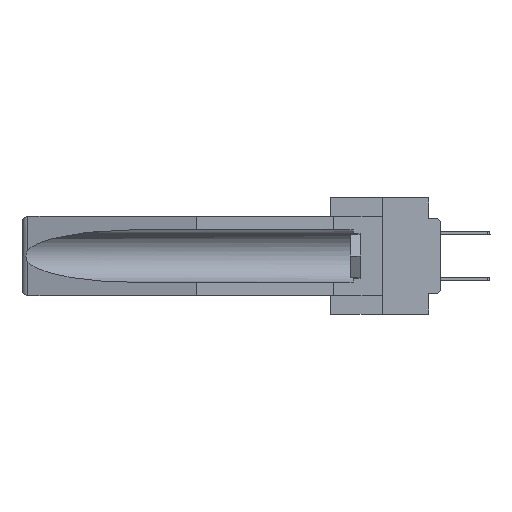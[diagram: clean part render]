
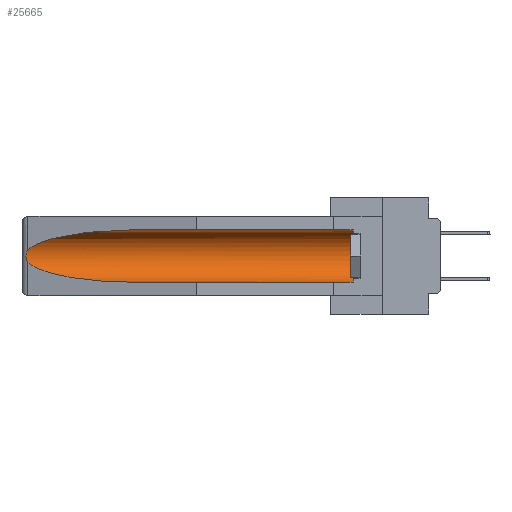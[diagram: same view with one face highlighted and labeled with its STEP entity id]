
A CAD part, left-side view. The second image highlights one B-rep face of the part: STEP entity #25665.
In plain terms, the highlighted cylindrical face has radius 2.857 mm (diameter 5.715 mm), a partial arc.
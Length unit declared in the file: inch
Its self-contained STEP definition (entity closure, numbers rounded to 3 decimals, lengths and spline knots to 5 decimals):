
#781 = DIRECTION ( 'NONE',  ( 0., 1., 0. ) ) ;
#2296 = B_SPLINE_CURVE_WITH_KNOTS ( 'NONE', 3,
 ( #31981, #20603, #7897, #35157, #5261, #5148, #26919, #10725, #21651, #21196 ),
 .UNSPECIFIED., .F., .F.,
 ( 4, 2, 2, 2, 4 ),
 ( 0., 0.00029, 0.00058, 0.00087, 0.00117 ),
 .UNSPECIFIED. ) ;
#3441 = CARTESIAN_POINT ( 'NONE',  ( 0.26537, 1.52718, -0.19328 ) ) ;
#3560 = CARTESIAN_POINT ( 'NONE',  ( 0.21114, 1.30732, -0.284 ) ) ;
#3565 = LINE ( 'NONE', #33325, #16690 ) ;
#5086 = VERTEX_POINT ( 'NONE', #35003 ) ;
#5148 = CARTESIAN_POINT ( 'NONE',  ( 0.2675, 1.53308, -0.17534 ) ) ;
#5261 = CARTESIAN_POINT ( 'NONE',  ( 0.2675, 1.53308, -0.16763 ) ) ;
#6193 = CARTESIAN_POINT ( 'NONE',  ( 0.25451, 1.48313, -0.24835 ) ) ;
#6838 = CARTESIAN_POINT ( 'NONE',  ( 0.155, 0.126, -0.1715 ) ) ;
#7038 = DIRECTION ( 'NONE',  ( 0., 1., 0. ) ) ;
#7275 = DIRECTION ( 'NONE',  ( 0., 0., 1. ) ) ;
#7372 = CARTESIAN_POINT ( 'NONE',  ( 0.26537, 1.52718, -0.19328 ) ) ;
#7897 = CARTESIAN_POINT ( 'NONE',  ( 0.26654, 1.53092, -0.15636 ) ) ;
#8513 = VERTEX_POINT ( 'NONE', #11826 ) ;
#10003 = CIRCLE ( 'NONE', #25782, 0.1125 ) ;
#10067 = ORIENTED_EDGE ( 'NONE', *, *, #34337, .T. ) ;
#10092 = CARTESIAN_POINT ( 'NONE',  ( 0.155, -0.30754, -0.1715 ) ) ;
#10140 = VECTOR ( 'NONE', #12170, 39.37008 ) ;
#10193 =( BOUNDED_CURVE ( )  B_SPLINE_CURVE ( 3, ( #3441, #6193, #3560, #12020 ),
 .UNSPECIFIED., .F., .F. ) 
 B_SPLINE_CURVE_WITH_KNOTS ( ( 4, 4 ),
 ( 0.1948, 1.5708 ),
 .UNSPECIFIED. ) 
 CURVE ( )  GEOMETRIC_REPRESENTATION_ITEM ( )  RATIONAL_B_SPLINE_CURVE ( ( 1., 0.848, 0.848, 1. ) ) 
 REPRESENTATION_ITEM ( '' )  );
#10725 = CARTESIAN_POINT ( 'NONE',  ( 0.26655, 1.53094, -0.18657 ) ) ;
#11826 = CARTESIAN_POINT ( 'NONE',  ( 0.155, 1.07973, -0.059 ) ) ;
#12020 = CARTESIAN_POINT ( 'NONE',  ( 0.155, 1.07973, -0.284 ) ) ;
#12170 = DIRECTION ( 'NONE',  ( 0., 1., 0. ) ) ;
#12618 = EDGE_LOOP ( 'NONE', ( #10067, #15345, #19010, #19520, #24973, #12813 ) ) ;
#12813 = ORIENTED_EDGE ( 'NONE', *, *, #26902, .T. ) ;
#13822 =( BOUNDED_CURVE ( )  B_SPLINE_CURVE ( 3, ( #18203, #20473, #28672, #17851 ),
 .UNSPECIFIED., .F., .F. ) 
 B_SPLINE_CURVE_WITH_KNOTS ( ( 4, 4 ),
 ( 4.71239, 6.08839 ),
 .UNSPECIFIED. ) 
 CURVE ( )  GEOMETRIC_REPRESENTATION_ITEM ( )  RATIONAL_B_SPLINE_CURVE ( ( 1., 0.848, 0.848, 1. ) ) 
 REPRESENTATION_ITEM ( '' )  );
#13954 = EDGE_CURVE ( 'NONE', #5086, #28427, #10003, .T. ) ;
#14765 = VERTEX_POINT ( 'NONE', #23408 ) ;
#14790 = LINE ( 'NONE', #26214, #10140 ) ;
#15345 = ORIENTED_EDGE ( 'NONE', *, *, #29674, .T. ) ;
#16668 = FACE_OUTER_BOUND ( 'NONE', #12618, .T. ) ;
#16690 = VECTOR ( 'NONE', #781, 39.37008 ) ;
#16967 = CARTESIAN_POINT ( 'NONE',  ( 0.155, 1.07973, -0.284 ) ) ;
#17052 = DIRECTION ( 'NONE',  ( 0., 0., 1. ) ) ;
#17851 = CARTESIAN_POINT ( 'NONE',  ( 0.26537, 1.52718, -0.14972 ) ) ;
#17987 = CYLINDRICAL_SURFACE ( 'NONE', #22239, 0.1125 ) ;
#18203 = CARTESIAN_POINT ( 'NONE',  ( 0.155, 1.07973, -0.059 ) ) ;
#19010 = ORIENTED_EDGE ( 'NONE', *, *, #29144, .T. ) ;
#19520 = ORIENTED_EDGE ( 'NONE', *, *, #32947, .F. ) ;
#20473 = CARTESIAN_POINT ( 'NONE',  ( 0.21114, 1.30732, -0.059 ) ) ;
#20603 = CARTESIAN_POINT ( 'NONE',  ( 0.26597, 1.52961, -0.15275 ) ) ;
#21196 = CARTESIAN_POINT ( 'NONE',  ( 0.26537, 1.52718, -0.19328 ) ) ;
#21651 = CARTESIAN_POINT ( 'NONE',  ( 0.26597, 1.5296, -0.19026 ) ) ;
#22239 = AXIS2_PLACEMENT_3D ( 'NONE', #10092, #7038, #7275 ) ;
#22422 = DIRECTION ( 'NONE',  ( 0., -1., 0. ) ) ;
#23408 = CARTESIAN_POINT ( 'NONE',  ( 0.26537, 1.52718, -0.14972 ) ) ;
#24973 = ORIENTED_EDGE ( 'NONE', *, *, #13954, .T. ) ;
#25665 = ADVANCED_FACE ( 'NONE', ( #16668 ), #17987, .F. ) ;
#25782 = AXIS2_PLACEMENT_3D ( 'NONE', #6838, #22422, #17052 ) ;
#26214 = CARTESIAN_POINT ( 'NONE',  ( 0.155, -0.30754, -0.059 ) ) ;
#26902 = EDGE_CURVE ( 'NONE', #28427, #8513, #14790, .T. ) ;
#26919 = CARTESIAN_POINT ( 'NONE',  ( 0.2673, 1.53269, -0.17917 ) ) ;
#27284 = VERTEX_POINT ( 'NONE', #16967 ) ;
#28427 = VERTEX_POINT ( 'NONE', #35076 ) ;
#28672 = CARTESIAN_POINT ( 'NONE',  ( 0.25451, 1.48313, -0.09465 ) ) ;
#29144 = EDGE_CURVE ( 'NONE', #29353, #27284, #10193, .T. ) ;
#29353 = VERTEX_POINT ( 'NONE', #7372 ) ;
#29674 = EDGE_CURVE ( 'NONE', #14765, #29353, #2296, .T. ) ;
#31981 = CARTESIAN_POINT ( 'NONE',  ( 0.26537, 1.52718, -0.14972 ) ) ;
#32947 = EDGE_CURVE ( 'NONE', #5086, #27284, #3565, .T. ) ;
#33325 = CARTESIAN_POINT ( 'NONE',  ( 0.155, -0.30754, -0.284 ) ) ;
#34337 = EDGE_CURVE ( 'NONE', #8513, #14765, #13822, .T. ) ;
#35003 = CARTESIAN_POINT ( 'NONE',  ( 0.155, 0.126, -0.284 ) ) ;
#35076 = CARTESIAN_POINT ( 'NONE',  ( 0.155, 0.126, -0.059 ) ) ;
#35157 = CARTESIAN_POINT ( 'NONE',  ( 0.2673, 1.5327, -0.16383 ) ) ;
